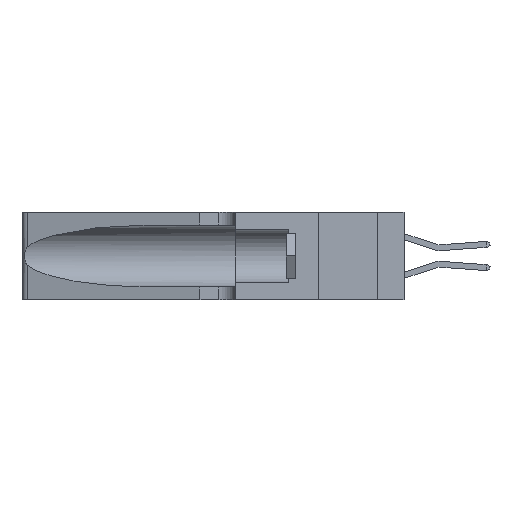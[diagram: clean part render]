
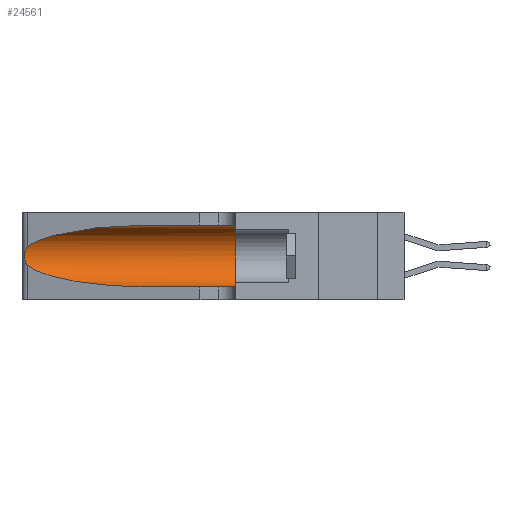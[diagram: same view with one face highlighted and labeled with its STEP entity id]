
A CAD part, left-side view. The second image highlights one B-rep face of the part: STEP entity #24561.
In plain terms, the highlighted cylindrical face has radius 3.308 mm (diameter 6.617 mm), a partial arc.
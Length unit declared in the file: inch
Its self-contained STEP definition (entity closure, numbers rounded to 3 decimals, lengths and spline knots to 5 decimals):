
#905 = VERTEX_POINT ( 'NONE', #31228 ) ;
#1075 = CIRCLE ( 'NONE', #24931, 0.13025 ) ;
#3100 = EDGE_CURVE ( 'NONE', #22015, #16672, #35585, .T. ) ;
#5009 = CARTESIAN_POINT ( 'NONE',  ( 0.1305, 0.72297, 0.31525 ) ) ;
#5982 = CARTESIAN_POINT ( 'NONE',  ( 0.26075, 1.23896, 0.19203 ) ) ;
#6266 = CARTESIAN_POINT ( 'NONE',  ( 0.25789, 1.23486, 0.15765 ) ) ;
#6426 = CARTESIAN_POINT ( 'NONE',  ( 0.1305, 1.61858, 0.31525 ) ) ;
#7004 = VERTEX_POINT ( 'NONE', #8356 ) ;
#8356 = CARTESIAN_POINT ( 'NONE',  ( 0.1305, 0.35, 0.31525 ) ) ;
#8444 = EDGE_CURVE ( 'NONE', #8785, #29050, #31858, .T. ) ;
#8486 = ORIENTED_EDGE ( 'NONE', *, *, #42608, .T. ) ;
#8785 = VERTEX_POINT ( 'NONE', #26072 ) ;
#9035 = CARTESIAN_POINT ( 'NONE',  ( 0.1305, 0.72297, 0.05475 ) ) ;
#9631 = CARTESIAN_POINT ( 'NONE',  ( 0.1305, 1.61858, 0.05475 ) ) ;
#11116 = CARTESIAN_POINT ( 'NONE',  ( 0.25487, 1.22718, 0.14631 ) ) ;
#11178 = CYLINDRICAL_SURFACE ( 'NONE', #17234, 0.13025 ) ;
#12193 = EDGE_LOOP ( 'NONE', ( #13603, #8486, #40274, #43019, #19372, #18888 ) ) ;
#13392 = DIRECTION ( 'NONE',  ( 0., 0., -1. ) ) ;
#13603 = ORIENTED_EDGE ( 'NONE', *, *, #8444, .T. ) ;
#14508 = CARTESIAN_POINT ( 'NONE',  ( 0.2373, 1.15595, 0.08982 ) ) ;
#16672 = VERTEX_POINT ( 'NONE', #34943 ) ;
#17179 = CARTESIAN_POINT ( 'NONE',  ( 0.25487, 1.22718, 0.14631 ) ) ;
#17234 = AXIS2_PLACEMENT_3D ( 'NONE', #20728, #30329, #13392 ) ;
#17311 = CARTESIAN_POINT ( 'NONE',  ( 0.1305, 0.35, 0.185 ) ) ;
#18225 = EDGE_CURVE ( 'NONE', #16672, #905, #21791, .T. ) ;
#18888 = ORIENTED_EDGE ( 'NONE', *, *, #32507, .F. ) ;
#19243 = CARTESIAN_POINT ( 'NONE',  ( 0.25639, 1.23186, 0.15144 ) ) ;
#19372 = ORIENTED_EDGE ( 'NONE', *, *, #30338, .F. ) ;
#19513 = CARTESIAN_POINT ( 'NONE',  ( 0.26075, 1.23896, 0.178 ) ) ;
#19817 = CARTESIAN_POINT ( 'NONE',  ( 0.25555, 1.22993, 0.14849 ) ) ;
#20728 = CARTESIAN_POINT ( 'NONE',  ( 0.1305, 1.61858, 0.185 ) ) ;
#21319 = CARTESIAN_POINT ( 'NONE',  ( 0.2373, 1.15595, 0.28018 ) ) ;
#21791 = LINE ( 'NONE', #9631, #42113 ) ;
#22015 = VERTEX_POINT ( 'NONE', #17179 ) ;
#24031 = DIRECTION ( 'NONE',  ( 0., 1., 0. ) ) ;
#24561 = ADVANCED_FACE ( 'NONE', ( #39869 ), #11178, .F. ) ;
#24931 = AXIS2_PLACEMENT_3D ( 'NONE', #17311, #24031, #35833 ) ;
#25941 = CARTESIAN_POINT ( 'NONE',  ( 0.25487, 1.22718, 0.22369 ) ) ;
#26072 = CARTESIAN_POINT ( 'NONE',  ( 0.1305, 0.72297, 0.31525 ) ) ;
#26213 = CARTESIAN_POINT ( 'NONE',  ( 0.25854, 1.2359, 0.20912 ) ) ;
#26367 = CARTESIAN_POINT ( 'NONE',  ( 0.25787, 1.23484, 0.2124 ) ) ;
#27434 = LINE ( 'NONE', #6426, #35788 ) ;
#29050 = VERTEX_POINT ( 'NONE', #38840 ) ;
#29302 = CARTESIAN_POINT ( 'NONE',  ( 0.25487, 1.22718, 0.14631 ) ) ;
#30329 = DIRECTION ( 'NONE',  ( 0., -1., 0. ) ) ;
#30338 = EDGE_CURVE ( 'NONE', #7004, #905, #1075, .T. ) ;
#31228 = CARTESIAN_POINT ( 'NONE',  ( 0.1305, 0.35, 0.05475 ) ) ;
#31548 = CARTESIAN_POINT ( 'NONE',  ( 0.25487, 1.22718, 0.22369 ) ) ;
#31858 =( BOUNDED_CURVE ( )  B_SPLINE_CURVE ( 3, ( #5009, #41265, #21319, #31548 ),
 .UNSPECIFIED., .F., .T. ) 
 B_SPLINE_CURVE_WITH_KNOTS ( ( 4, 4 ),
 ( 1.5708, 2.84003 ),
 .UNSPECIFIED. ) 
 CURVE ( )  GEOMETRIC_REPRESENTATION_ITEM ( )  RATIONAL_B_SPLINE_CURVE ( ( 1., 0.87, 0.87, 1. ) ) 
 REPRESENTATION_ITEM ( '' )  );
#32507 = EDGE_CURVE ( 'NONE', #8785, #7004, #27434, .T. ) ;
#32509 = CARTESIAN_POINT ( 'NONE',  ( 0.26017, 1.23833, 0.17102 ) ) ;
#33860 = DIRECTION ( 'NONE',  ( 0., -1., 0. ) ) ;
#34943 = CARTESIAN_POINT ( 'NONE',  ( 0.1305, 0.72297, 0.05475 ) ) ;
#35585 =( BOUNDED_CURVE ( )  B_SPLINE_CURVE ( 3, ( #11116, #14508, #38010, #9035 ),
 .UNSPECIFIED., .F., .F. ) 
 B_SPLINE_CURVE_WITH_KNOTS ( ( 4, 4 ),
 ( 3.44316, 4.71239 ),
 .UNSPECIFIED. ) 
 CURVE ( )  GEOMETRIC_REPRESENTATION_ITEM ( )  RATIONAL_B_SPLINE_CURVE ( ( 1., 0.87, 0.87, 1. ) ) 
 REPRESENTATION_ITEM ( '' )  );
#35788 = VECTOR ( 'NONE', #36747, 39.37008 ) ;
#35833 = DIRECTION ( 'NONE',  ( 0., 0., 1. ) ) ;
#35872 = CARTESIAN_POINT ( 'NONE',  ( 0.26018, 1.23835, 0.19895 ) ) ;
#36304 = CARTESIAN_POINT ( 'NONE',  ( 0.25555, 1.22994, 0.2215 ) ) ;
#36747 = DIRECTION ( 'NONE',  ( 0., -1., 0. ) ) ;
#38010 = CARTESIAN_POINT ( 'NONE',  ( 0.18966, 0.96281, 0.05475 ) ) ;
#38840 = CARTESIAN_POINT ( 'NONE',  ( 0.25487, 1.22718, 0.22369 ) ) ;
#39774 = CARTESIAN_POINT ( 'NONE',  ( 0.25639, 1.23184, 0.21858 ) ) ;
#39869 = FACE_OUTER_BOUND ( 'NONE', #12193, .T. ) ;
#40274 = ORIENTED_EDGE ( 'NONE', *, *, #3100, .T. ) ;
#41265 = CARTESIAN_POINT ( 'NONE',  ( 0.18966, 0.96281, 0.31525 ) ) ;
#41994 = B_SPLINE_CURVE_WITH_KNOTS ( 'NONE', 3,
 ( #25941, #36304, #39774, #26367, #26213, #35872, #5982, #19513, #32509, #43132, #6266, #19243, #19817, #29302 ),
 .UNSPECIFIED., .F., .F.,
 ( 4, 2, 2, 2, 2, 2, 4 ),
 ( 0., 0.00027, 0.00053, 0.00107, 0.0016, 0.00187, 0.00214 ),
 .UNSPECIFIED. ) ;
#42113 = VECTOR ( 'NONE', #33860, 39.37008 ) ;
#42608 = EDGE_CURVE ( 'NONE', #29050, #22015, #41994, .T. ) ;
#43019 = ORIENTED_EDGE ( 'NONE', *, *, #18225, .T. ) ;
#43132 = CARTESIAN_POINT ( 'NONE',  ( 0.25856, 1.23593, 0.16098 ) ) ;
